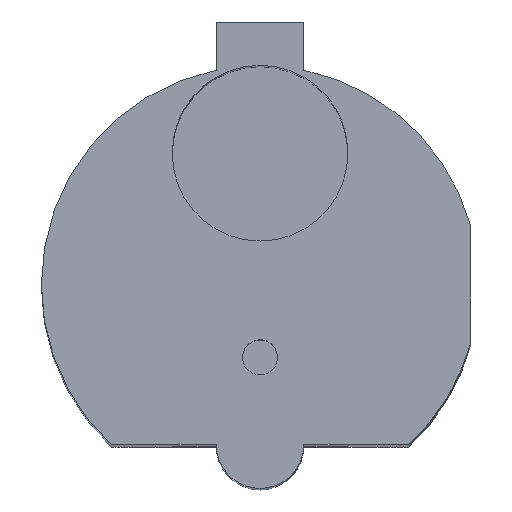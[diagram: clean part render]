
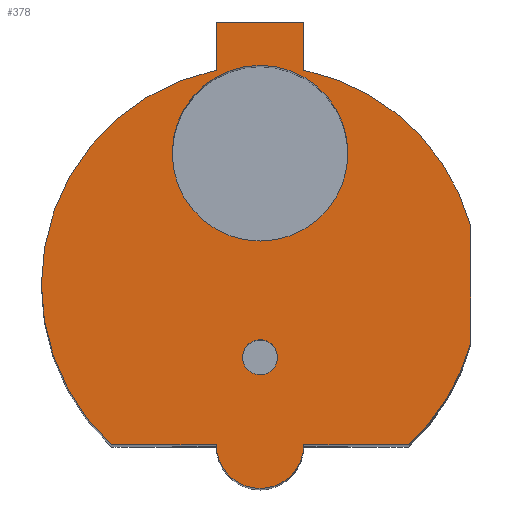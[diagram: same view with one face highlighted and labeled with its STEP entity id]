
A CAD part, top view. The second image highlights one B-rep face of the part: STEP entity #378.
In plain terms, the highlighted planar face has unit normal (0, 0, 1).
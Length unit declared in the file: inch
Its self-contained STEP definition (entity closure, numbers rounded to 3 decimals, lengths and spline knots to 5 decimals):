
#13 = DIRECTION ( 'NONE',  ( 0., 0., 1. ) ) ;
#15 = CARTESIAN_POINT ( 'NONE',  ( 0.7222, 0.2023, 2.9 ) ) ;
#19 = VERTEX_POINT ( 'NONE', #1239 ) ;
#29 = EDGE_CURVE ( 'NONE', #174, #571, #712, .T. ) ;
#33 = AXIS2_PLACEMENT_3D ( 'NONE', #330, #987, #886 ) ;
#40 = CARTESIAN_POINT ( 'NONE',  ( 0., -0.25, 2.9 ) ) ;
#46 = AXIS2_PLACEMENT_3D ( 'NONE', #1023, #13, #1111 ) ;
#67 = FACE_OUTER_BOUND ( 'NONE', #1208, .T. ) ;
#78 = AXIS2_PLACEMENT_3D ( 'NONE', #862, #978, #202 ) ;
#79 = CARTESIAN_POINT ( 'NONE',  ( 0.06, -0.25, 2.9 ) ) ;
#80 = EDGE_CURVE ( 'NONE', #136, #894, #1309, .T. ) ;
#82 = DIRECTION ( 'NONE',  ( 1., 0., 0. ) ) ;
#97 = VECTOR ( 'NONE', #1200, 39.37008 ) ;
#116 = LINE ( 'NONE', #654, #1187 ) ;
#119 = ORIENTED_EDGE ( 'NONE', *, *, #500, .F. ) ;
#127 = CARTESIAN_POINT ( 'NONE',  ( 0., 0.45, 2.9 ) ) ;
#128 = EDGE_CURVE ( 'NONE', #928, #1326, #959, .T. ) ;
#132 = DIRECTION ( 'NONE',  ( 1., 0., 0. ) ) ;
#136 = VERTEX_POINT ( 'NONE', #1227 ) ;
#151 = CARTESIAN_POINT ( 'NONE',  ( -0.15, 0.73485, 2.9 ) ) ;
#168 = AXIS2_PLACEMENT_3D ( 'NONE', #127, #776, #132 ) ;
#174 = VERTEX_POINT ( 'NONE', #572 ) ;
#200 = AXIS2_PLACEMENT_3D ( 'NONE', #1298, #844, #82 ) ;
#202 = DIRECTION ( 'NONE',  ( 1., 0., 0. ) ) ;
#204 = ORIENTED_EDGE ( 'NONE', *, *, #579, .T. ) ;
#207 = ORIENTED_EDGE ( 'NONE', *, *, #456, .F. ) ;
#232 = LINE ( 'NONE', #612, #97 ) ;
#269 = CIRCLE ( 'NONE', #664, 0.30131 ) ;
#280 = AXIS2_PLACEMENT_3D ( 'NONE', #1055, #1282, #718 ) ;
#299 = AXIS2_PLACEMENT_3D ( 'NONE', #1029, #574, #668 ) ;
#301 = EDGE_CURVE ( 'NONE', #855, #136, #401, .T. ) ;
#330 = CARTESIAN_POINT ( 'NONE',  ( 0., 0., 2.9 ) ) ;
#338 = VERTEX_POINT ( 'NONE', #710 ) ;
#350 = FACE_BOUND ( 'NONE', #1145, .T. ) ;
#352 = VERTEX_POINT ( 'NONE', #1279 ) ;
#357 = VECTOR ( 'NONE', #545, 39.37008 ) ;
#376 = ORIENTED_EDGE ( 'NONE', *, *, #1306, .F. ) ;
#378 = ADVANCED_FACE ( 'NONE', ( #1323, #350, #67 ), #1291, .T. ) ;
#380 = AXIS2_PLACEMENT_3D ( 'NONE', #40, #1131, #1144 ) ;
#385 = ORIENTED_EDGE ( 'NONE', *, *, #1007, .F. ) ;
#401 = CIRCLE ( 'NONE', #1036, 0.75 ) ;
#412 = EDGE_CURVE ( 'NONE', #571, #174, #269, .T. ) ;
#418 = DIRECTION ( 'NONE',  ( 0., 1., 0. ) ) ;
#426 = CARTESIAN_POINT ( 'NONE',  ( -0.15, -0.55, 2.9 ) ) ;
#456 = EDGE_CURVE ( 'NONE', #1284, #19, #232, .T. ) ;
#472 = EDGE_CURVE ( 'NONE', #1173, #19, #798, .T. ) ;
#491 = DIRECTION ( 'NONE',  ( 1., 0., 0. ) ) ;
#499 = ORIENTED_EDGE ( 'NONE', *, *, #301, .T. ) ;
#500 = EDGE_CURVE ( 'NONE', #338, #352, #1154, .T. ) ;
#519 = CIRCLE ( 'NONE', #33, 0.75 ) ;
#520 = ORIENTED_EDGE ( 'NONE', *, *, #128, .T. ) ;
#530 = ORIENTED_EDGE ( 'NONE', *, *, #472, .T. ) ;
#534 = CARTESIAN_POINT ( 'NONE',  ( -0.15, 0., 2.9 ) ) ;
#545 = DIRECTION ( 'NONE',  ( 0., -1., 0. ) ) ;
#571 = VERTEX_POINT ( 'NONE', #1104 ) ;
#572 = CARTESIAN_POINT ( 'NONE',  ( 0.30131, 0.45, 2.9 ) ) ;
#574 = DIRECTION ( 'NONE',  ( 0., 0., 1. ) ) ;
#579 = EDGE_CURVE ( 'NONE', #1210, #1173, #116, .T. ) ;
#588 = CARTESIAN_POINT ( 'NONE',  ( 0., 0., 2.9 ) ) ;
#607 = CARTESIAN_POINT ( 'NONE',  ( 0., -0.55, 2.9 ) ) ;
#608 = ORIENTED_EDGE ( 'NONE', *, *, #412, .F. ) ;
#612 = CARTESIAN_POINT ( 'NONE',  ( 0.15, 0., 2.9 ) ) ;
#620 = CARTESIAN_POINT ( 'NONE',  ( 0., -0.55, 2.9 ) ) ;
#654 = CARTESIAN_POINT ( 'NONE',  ( 0.7222, 0., 2.9 ) ) ;
#661 = CARTESIAN_POINT ( 'NONE',  ( 0.7222, -0.2023, 2.9 ) ) ;
#664 = AXIS2_PLACEMENT_3D ( 'NONE', #860, #957, #846 ) ;
#668 = DIRECTION ( 'NONE',  ( 1., 0., 0. ) ) ;
#677 = CIRCLE ( 'NONE', #78, 0.06 ) ;
#689 = CARTESIAN_POINT ( 'NONE',  ( -0.06, -0.25, 2.9 ) ) ;
#710 = CARTESIAN_POINT ( 'NONE',  ( 0.5099, -0.55, 2.9 ) ) ;
#712 = CIRCLE ( 'NONE', #168, 0.30131 ) ;
#718 = DIRECTION ( 'NONE',  ( 1., 0., 0. ) ) ;
#732 = ORIENTED_EDGE ( 'NONE', *, *, #1217, .T. ) ;
#768 = ORIENTED_EDGE ( 'NONE', *, *, #1203, .T. ) ;
#776 = DIRECTION ( 'NONE',  ( 0., 0., 1. ) ) ;
#786 = VECTOR ( 'NONE', #1129, 39.37008 ) ;
#798 = CIRCLE ( 'NONE', #200, 0.75 ) ;
#844 = DIRECTION ( 'NONE',  ( 0., 0., 1. ) ) ;
#846 = DIRECTION ( 'NONE',  ( 1., 0., 0. ) ) ;
#855 = VERTEX_POINT ( 'NONE', #151 ) ;
#859 = CIRCLE ( 'NONE', #299, 0.15 ) ;
#860 = CARTESIAN_POINT ( 'NONE',  ( 0., 0.45, 2.9 ) ) ;
#862 = CARTESIAN_POINT ( 'NONE',  ( 0., -0.25, 2.9 ) ) ;
#886 = DIRECTION ( 'NONE',  ( 1., 0., 0. ) ) ;
#894 = VERTEX_POINT ( 'NONE', #1165 ) ;
#928 = VERTEX_POINT ( 'NONE', #79 ) ;
#952 = DIRECTION ( 'NONE',  ( -1., 0., 0. ) ) ;
#953 = DIRECTION ( 'NONE',  ( 0., 0., 1. ) ) ;
#957 = DIRECTION ( 'NONE',  ( 0., 0., 1. ) ) ;
#959 = CIRCLE ( 'NONE', #380, 0.06 ) ;
#978 = DIRECTION ( 'NONE',  ( 0., 0., -1. ) ) ;
#980 = VERTEX_POINT ( 'NONE', #1052 ) ;
#987 = DIRECTION ( 'NONE',  ( 0., 0., 1. ) ) ;
#1007 = EDGE_CURVE ( 'NONE', #1214, #894, #1384, .T. ) ;
#1023 = CARTESIAN_POINT ( 'NONE',  ( 0., 0., 2.9 ) ) ;
#1029 = CARTESIAN_POINT ( 'NONE',  ( 0., -0.55, 2.9 ) ) ;
#1036 = AXIS2_PLACEMENT_3D ( 'NONE', #588, #953, #491 ) ;
#1052 = CARTESIAN_POINT ( 'NONE',  ( -0.15, 0.9, 2.9 ) ) ;
#1055 = CARTESIAN_POINT ( 'NONE',  ( 0., 0., 2.9 ) ) ;
#1076 = DIRECTION ( 'NONE',  ( -1., 0., 0. ) ) ;
#1080 = ORIENTED_EDGE ( 'NONE', *, *, #1296, .T. ) ;
#1088 = VECTOR ( 'NONE', #952, 39.37008 ) ;
#1104 = CARTESIAN_POINT ( 'NONE',  ( -0.30131, 0.45, 2.9 ) ) ;
#1107 = EDGE_CURVE ( 'NONE', #1326, #928, #677, .T. ) ;
#1111 = DIRECTION ( 'NONE',  ( 1., 0., 0. ) ) ;
#1129 = DIRECTION ( 'NONE',  ( 1., 0., 0. ) ) ;
#1131 = DIRECTION ( 'NONE',  ( 0., 0., -1. ) ) ;
#1144 = DIRECTION ( 'NONE',  ( 1., 0., 0. ) ) ;
#1145 = EDGE_LOOP ( 'NONE', ( #520, #1177 ) ) ;
#1154 = LINE ( 'NONE', #620, #1424 ) ;
#1165 = CARTESIAN_POINT ( 'NONE',  ( -0.5099, -0.55, 2.9 ) ) ;
#1173 = VERTEX_POINT ( 'NONE', #15 ) ;
#1177 = ORIENTED_EDGE ( 'NONE', *, *, #1107, .T. ) ;
#1187 = VECTOR ( 'NONE', #418, 39.37008 ) ;
#1200 = DIRECTION ( 'NONE',  ( 0., -1., 0. ) ) ;
#1203 = EDGE_CURVE ( 'NONE', #338, #1210, #519, .T. ) ;
#1208 = EDGE_LOOP ( 'NONE', ( #768, #204, #530, #207, #376, #732, #499, #1316, #385, #1080, #119 ) ) ;
#1210 = VERTEX_POINT ( 'NONE', #661 ) ;
#1214 = VERTEX_POINT ( 'NONE', #426 ) ;
#1217 = EDGE_CURVE ( 'NONE', #980, #855, #1286, .T. ) ;
#1227 = CARTESIAN_POINT ( 'NONE',  ( -0.75, 0., 2.9 ) ) ;
#1233 = ORIENTED_EDGE ( 'NONE', *, *, #29, .F. ) ;
#1239 = CARTESIAN_POINT ( 'NONE',  ( 0.15, 0.73485, 2.9 ) ) ;
#1279 = CARTESIAN_POINT ( 'NONE',  ( 0.15, -0.55, 2.9 ) ) ;
#1282 = DIRECTION ( 'NONE',  ( 0., 0., 1. ) ) ;
#1284 = VERTEX_POINT ( 'NONE', #1354 ) ;
#1286 = LINE ( 'NONE', #534, #357 ) ;
#1291 = PLANE ( 'NONE',  #280 ) ;
#1296 = EDGE_CURVE ( 'NONE', #1214, #352, #859, .T. ) ;
#1298 = CARTESIAN_POINT ( 'NONE',  ( 0., 0., 2.9 ) ) ;
#1306 = EDGE_CURVE ( 'NONE', #980, #1284, #1361, .T. ) ;
#1309 = CIRCLE ( 'NONE', #46, 0.75 ) ;
#1316 = ORIENTED_EDGE ( 'NONE', *, *, #80, .T. ) ;
#1323 = FACE_BOUND ( 'NONE', #1411, .T. ) ;
#1326 = VERTEX_POINT ( 'NONE', #689 ) ;
#1350 = CARTESIAN_POINT ( 'NONE',  ( 0., 0.9, 2.9 ) ) ;
#1354 = CARTESIAN_POINT ( 'NONE',  ( 0.15, 0.9, 2.9 ) ) ;
#1361 = LINE ( 'NONE', #1350, #786 ) ;
#1384 = LINE ( 'NONE', #607, #1088 ) ;
#1411 = EDGE_LOOP ( 'NONE', ( #1233, #608 ) ) ;
#1424 = VECTOR ( 'NONE', #1076, 39.37008 ) ;
